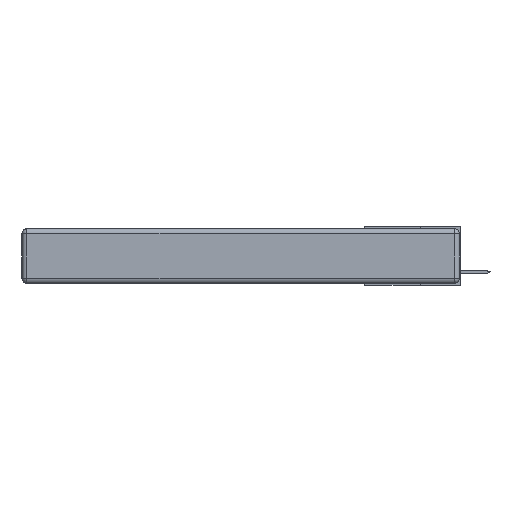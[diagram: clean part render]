
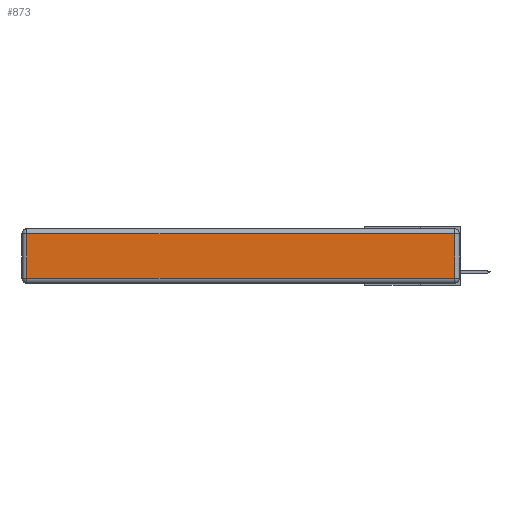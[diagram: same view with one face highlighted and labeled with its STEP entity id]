
A CAD part, left-side view. The second image highlights one B-rep face of the part: STEP entity #873.
In plain terms, the highlighted planar face has unit normal (-1, 0, 0).
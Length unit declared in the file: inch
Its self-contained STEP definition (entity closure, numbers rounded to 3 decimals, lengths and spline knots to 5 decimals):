
#717 = ORIENTED_EDGE ( 'NONE', *, *, #21118, .T. ) ;
#873 = ADVANCED_FACE ( 'NONE', ( #20416 ), #6400, .T. ) ;
#1238 = EDGE_CURVE ( 'NONE', #18954, #3523, #11160, .T. ) ;
#1251 = CARTESIAN_POINT ( 'NONE',  ( 0., 0.03, -0.03 ) ) ;
#2578 = DIRECTION ( 'NONE',  ( 0., 0., -1. ) ) ;
#2670 = CARTESIAN_POINT ( 'NONE',  ( 0., 0.03, -0.343 ) ) ;
#2885 = ORIENTED_EDGE ( 'NONE', *, *, #6697, .T. ) ;
#3034 = ORIENTED_EDGE ( 'NONE', *, *, #13907, .T. ) ;
#3035 = VECTOR ( 'NONE', #11054, 39.37008 ) ;
#3523 = VERTEX_POINT ( 'NONE', #13768 ) ;
#4241 = AXIS2_PLACEMENT_3D ( 'NONE', #6690, #5095, #18278 ) ;
#5095 = DIRECTION ( 'NONE',  ( -1., 0., 0. ) ) ;
#6400 = PLANE ( 'NONE',  #4241 ) ;
#6690 = CARTESIAN_POINT ( 'NONE',  ( 0., 0., -0.343 ) ) ;
#6697 = EDGE_CURVE ( 'NONE', #11242, #18954, #11743, .T. ) ;
#9356 = VECTOR ( 'NONE', #2578, 39.37008 ) ;
#10988 = DIRECTION ( 'NONE',  ( 0., -1., 0. ) ) ;
#11054 = DIRECTION ( 'NONE',  ( 0., 0., 1. ) ) ;
#11160 = LINE ( 'NONE', #15710, #9356 ) ;
#11236 = CARTESIAN_POINT ( 'NONE',  ( 0., 2.75, -0.03 ) ) ;
#11242 = VERTEX_POINT ( 'NONE', #1251 ) ;
#11417 = ORIENTED_EDGE ( 'NONE', *, *, #1238, .T. ) ;
#11526 = DIRECTION ( 'NONE',  ( 0., 1., 0. ) ) ;
#11743 = LINE ( 'NONE', #11236, #12527 ) ;
#12527 = VECTOR ( 'NONE', #11526, 39.37008 ) ;
#13302 = CARTESIAN_POINT ( 'NONE',  ( 0., 2.72, -0.03 ) ) ;
#13768 = CARTESIAN_POINT ( 'NONE',  ( 0., 2.72, -0.313 ) ) ;
#13907 = EDGE_CURVE ( 'NONE', #3523, #17568, #17044, .T. ) ;
#15490 = VECTOR ( 'NONE', #10988, 39.37008 ) ;
#15710 = CARTESIAN_POINT ( 'NONE',  ( 0., 2.72, -0.343 ) ) ;
#16103 = EDGE_LOOP ( 'NONE', ( #3034, #717, #2885, #11417 ) ) ;
#16262 = CARTESIAN_POINT ( 'NONE',  ( 0., 0.03, -0.313 ) ) ;
#17044 = LINE ( 'NONE', #17260, #15490 ) ;
#17260 = CARTESIAN_POINT ( 'NONE',  ( 0., 0., -0.313 ) ) ;
#17568 = VERTEX_POINT ( 'NONE', #16262 ) ;
#18278 = DIRECTION ( 'NONE',  ( 0., 0., 1. ) ) ;
#18954 = VERTEX_POINT ( 'NONE', #13302 ) ;
#20416 = FACE_OUTER_BOUND ( 'NONE', #16103, .T. ) ;
#20493 = LINE ( 'NONE', #2670, #3035 ) ;
#21118 = EDGE_CURVE ( 'NONE', #17568, #11242, #20493, .T. ) ;
